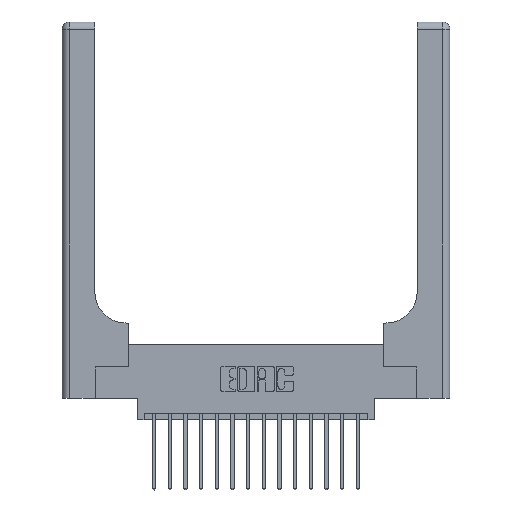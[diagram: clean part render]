
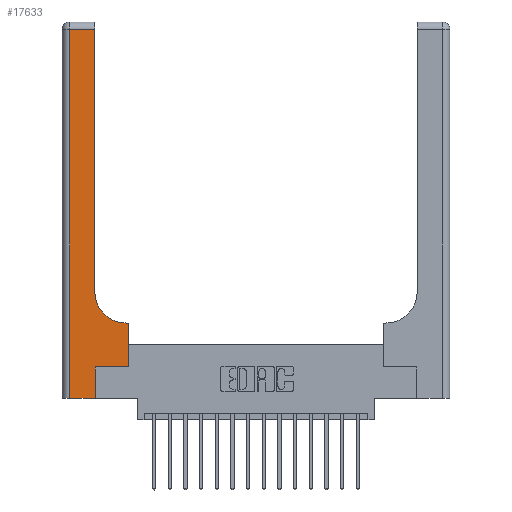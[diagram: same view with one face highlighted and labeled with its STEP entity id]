
A CAD part, top view. The second image highlights one B-rep face of the part: STEP entity #17633.
In plain terms, the highlighted planar face has unit normal (0, 0, 1).
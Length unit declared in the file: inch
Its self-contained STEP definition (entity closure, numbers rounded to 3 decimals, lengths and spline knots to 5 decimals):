
#601 = FACE_OUTER_BOUND ( 'NONE', #6753, .T. ) ;
#784 = ORIENTED_EDGE ( 'NONE', *, *, #7456, .T. ) ;
#905 = CARTESIAN_POINT ( 'NONE',  ( 0.26, 0.85, 0.37 ) ) ;
#1497 = DIRECTION ( 'NONE',  ( 0., 1., 0. ) ) ;
#1749 = VERTEX_POINT ( 'NONE', #5814 ) ;
#1808 = CARTESIAN_POINT ( 'NONE',  ( 0., 3., 0.37 ) ) ;
#2033 = DIRECTION ( 'NONE',  ( 0., 0., -1. ) ) ;
#2081 = EDGE_CURVE ( 'NONE', #1749, #13873, #3376, .T. ) ;
#2388 = VECTOR ( 'NONE', #5364, 39.37008 ) ;
#2511 = AXIS2_PLACEMENT_3D ( 'NONE', #1808, #3242, #13106 ) ;
#2592 = LINE ( 'NONE', #14563, #9664 ) ;
#2605 = EDGE_CURVE ( 'NONE', #10380, #7227, #10409, .T. ) ;
#2615 = LINE ( 'NONE', #3406, #13441 ) ;
#3024 = AXIS2_PLACEMENT_3D ( 'NONE', #10490, #2033, #11895 ) ;
#3242 = DIRECTION ( 'NONE',  ( 0., 0., -1. ) ) ;
#3366 = CARTESIAN_POINT ( 'NONE',  ( 0., 2.94, 0.37 ) ) ;
#3376 = LINE ( 'NONE', #17779, #17931 ) ;
#3406 = CARTESIAN_POINT ( 'NONE',  ( 0.265, 0., 0.37 ) ) ;
#3864 = CARTESIAN_POINT ( 'NONE',  ( 0.265, 0.25, 0.37 ) ) ;
#4759 = DIRECTION ( 'NONE',  ( 1., 0., 0. ) ) ;
#4936 = ORIENTED_EDGE ( 'NONE', *, *, #11563, .T. ) ;
#4983 = VERTEX_POINT ( 'NONE', #9369 ) ;
#5056 = VERTEX_POINT ( 'NONE', #9547 ) ;
#5364 = DIRECTION ( 'NONE',  ( 0., -1., 0. ) ) ;
#5539 = LINE ( 'NONE', #11365, #5974 ) ;
#5814 = CARTESIAN_POINT ( 'NONE',  ( 0.528, 0.6, 0.37 ) ) ;
#5974 = VECTOR ( 'NONE', #1497, 39.37008 ) ;
#6206 = VECTOR ( 'NONE', #16153, 39.37008 ) ;
#6594 = DIRECTION ( 'NONE',  ( -1., 0., 0. ) ) ;
#6639 = CIRCLE ( 'NONE', #3024, 0.25 ) ;
#6753 = EDGE_LOOP ( 'NONE', ( #15080, #13565, #17744, #14416, #4936, #13351, #784, #7316, #13311 ) ) ;
#6881 = CARTESIAN_POINT ( 'NONE',  ( 0.51, 0.6, 0.37 ) ) ;
#7227 = VERTEX_POINT ( 'NONE', #11963 ) ;
#7316 = ORIENTED_EDGE ( 'NONE', *, *, #2081, .T. ) ;
#7456 = EDGE_CURVE ( 'NONE', #4983, #1749, #13372, .T. ) ;
#8031 = VERTEX_POINT ( 'NONE', #905 ) ;
#8861 = VERTEX_POINT ( 'NONE', #11403 ) ;
#9133 = CARTESIAN_POINT ( 'NONE',  ( 0., 0., 0.37 ) ) ;
#9369 = CARTESIAN_POINT ( 'NONE',  ( 0.528, 0.25, 0.37 ) ) ;
#9459 = LINE ( 'NONE', #13834, #2388 ) ;
#9547 = CARTESIAN_POINT ( 'NONE',  ( 0.26, 2.94, 0.37 ) ) ;
#9664 = VECTOR ( 'NONE', #4759, 39.37008 ) ;
#9919 = EDGE_CURVE ( 'NONE', #13873, #8031, #6639, .T. ) ;
#10266 = PLANE ( 'NONE',  #2511 ) ;
#10380 = VERTEX_POINT ( 'NONE', #13124 ) ;
#10409 = LINE ( 'NONE', #9133, #6206 ) ;
#10490 = CARTESIAN_POINT ( 'NONE',  ( 0.51, 0.85, 0.37 ) ) ;
#11039 = DIRECTION ( 'NONE',  ( 0., 1., 0. ) ) ;
#11268 = LINE ( 'NONE', #3366, #15011 ) ;
#11365 = CARTESIAN_POINT ( 'NONE',  ( 0.26, 3., 0.37 ) ) ;
#11403 = CARTESIAN_POINT ( 'NONE',  ( 0.06, 2.94, 0.37 ) ) ;
#11563 = EDGE_CURVE ( 'NONE', #7227, #15510, #2615, .T. ) ;
#11806 = EDGE_CURVE ( 'NONE', #8861, #10380, #9459, .T. ) ;
#11844 = DIRECTION ( 'NONE',  ( 0., 1., 0. ) ) ;
#11895 = DIRECTION ( 'NONE',  ( 1., 0., 0. ) ) ;
#11963 = CARTESIAN_POINT ( 'NONE',  ( 0.265, 0., 0.37 ) ) ;
#12463 = CARTESIAN_POINT ( 'NONE',  ( 0.528, 0.25, 0.37 ) ) ;
#13106 = DIRECTION ( 'NONE',  ( -1., 0., 0. ) ) ;
#13124 = CARTESIAN_POINT ( 'NONE',  ( 0.06, 0., 0.37 ) ) ;
#13311 = ORIENTED_EDGE ( 'NONE', *, *, #9919, .T. ) ;
#13351 = ORIENTED_EDGE ( 'NONE', *, *, #17711, .T. ) ;
#13372 = LINE ( 'NONE', #12463, #16676 ) ;
#13441 = VECTOR ( 'NONE', #11844, 39.37008 ) ;
#13565 = ORIENTED_EDGE ( 'NONE', *, *, #14631, .T. ) ;
#13834 = CARTESIAN_POINT ( 'NONE',  ( 0.06, 3., 0.37 ) ) ;
#13873 = VERTEX_POINT ( 'NONE', #6881 ) ;
#14416 = ORIENTED_EDGE ( 'NONE', *, *, #2605, .T. ) ;
#14529 = EDGE_CURVE ( 'NONE', #8031, #5056, #5539, .T. ) ;
#14563 = CARTESIAN_POINT ( 'NONE',  ( 0.265, 0.25, 0.37 ) ) ;
#14625 = DIRECTION ( 'NONE',  ( -1., 0., 0. ) ) ;
#14631 = EDGE_CURVE ( 'NONE', #5056, #8861, #11268, .T. ) ;
#15011 = VECTOR ( 'NONE', #14625, 39.37008 ) ;
#15080 = ORIENTED_EDGE ( 'NONE', *, *, #14529, .T. ) ;
#15510 = VERTEX_POINT ( 'NONE', #3864 ) ;
#16153 = DIRECTION ( 'NONE',  ( 1., 0., 0. ) ) ;
#16676 = VECTOR ( 'NONE', #11039, 39.37008 ) ;
#17633 = ADVANCED_FACE ( 'NONE', ( #601 ), #10266, .F. ) ;
#17711 = EDGE_CURVE ( 'NONE', #15510, #4983, #2592, .T. ) ;
#17744 = ORIENTED_EDGE ( 'NONE', *, *, #11806, .T. ) ;
#17779 = CARTESIAN_POINT ( 'NONE',  ( 0.26, 0.6, 0.37 ) ) ;
#17931 = VECTOR ( 'NONE', #6594, 39.37008 ) ;
